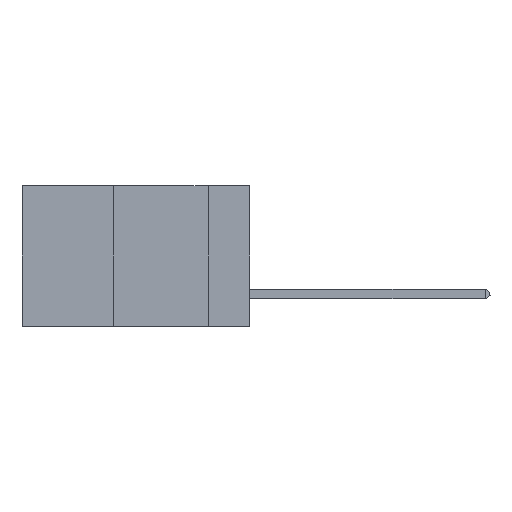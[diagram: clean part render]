
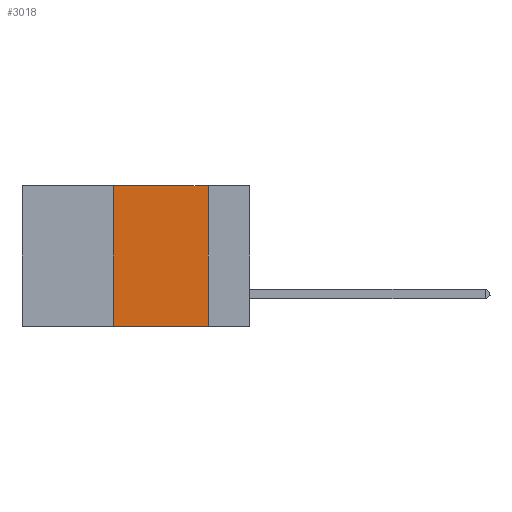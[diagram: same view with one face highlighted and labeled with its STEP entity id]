
A CAD part, left-side view. The second image highlights one B-rep face of the part: STEP entity #3018.
In plain terms, the highlighted planar face has unit normal (-1, 0, 0).
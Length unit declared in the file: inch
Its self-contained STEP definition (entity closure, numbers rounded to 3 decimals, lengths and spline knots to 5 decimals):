
#1226 = CARTESIAN_POINT ( 'NONE',  ( 0., 0.36, -0.37 ) ) ;
#2201 = ORIENTED_EDGE ( 'NONE', *, *, #19495, .F. ) ;
#3018 = ADVANCED_FACE ( 'NONE', ( #18363 ), #25612, .F. ) ;
#3512 = CARTESIAN_POINT ( 'NONE',  ( 0., 0.11, 0. ) ) ;
#3960 = CARTESIAN_POINT ( 'NONE',  ( 0., 0.6, 0. ) ) ;
#7002 = LINE ( 'NONE', #27579, #41238 ) ;
#7338 = DIRECTION ( 'NONE',  ( 0., -1., 0. ) ) ;
#7457 = LINE ( 'NONE', #19322, #32576 ) ;
#8779 = ORIENTED_EDGE ( 'NONE', *, *, #45104, .T. ) ;
#9401 = DIRECTION ( 'NONE',  ( 0., -1., 0. ) ) ;
#9418 = AXIS2_PLACEMENT_3D ( 'NONE', #3960, #40113, #14275 ) ;
#12452 = ORIENTED_EDGE ( 'NONE', *, *, #36533, .F. ) ;
#14275 = DIRECTION ( 'NONE',  ( 0., 0., -1. ) ) ;
#18363 = FACE_OUTER_BOUND ( 'NONE', #40844, .T. ) ;
#19003 = DIRECTION ( 'NONE',  ( 0., 0., 1. ) ) ;
#19322 = CARTESIAN_POINT ( 'NONE',  ( 0., 0.36, 0. ) ) ;
#19495 = EDGE_CURVE ( 'NONE', #38282, #29687, #7457, .T. ) ;
#21006 = CARTESIAN_POINT ( 'NONE',  ( 0., 0.11, -0.37 ) ) ;
#25612 = PLANE ( 'NONE',  #9418 ) ;
#26482 = LINE ( 'NONE', #39075, #32237 ) ;
#27579 = CARTESIAN_POINT ( 'NONE',  ( 0., 0.6, -0.37 ) ) ;
#29160 = CARTESIAN_POINT ( 'NONE',  ( 0., 0.6, 0. ) ) ;
#29687 = VERTEX_POINT ( 'NONE', #39628 ) ;
#32237 = VECTOR ( 'NONE', #42750, 39.37008 ) ;
#32412 = VERTEX_POINT ( 'NONE', #21006 ) ;
#32539 = ORIENTED_EDGE ( 'NONE', *, *, #43682, .F. ) ;
#32576 = VECTOR ( 'NONE', #19003, 39.37008 ) ;
#33911 = LINE ( 'NONE', #29160, #36169 ) ;
#36169 = VECTOR ( 'NONE', #7338, 39.37008 ) ;
#36533 = EDGE_CURVE ( 'NONE', #29687, #42153, #33911, .T. ) ;
#38282 = VERTEX_POINT ( 'NONE', #1226 ) ;
#39075 = CARTESIAN_POINT ( 'NONE',  ( 0., 0.11, 0. ) ) ;
#39628 = CARTESIAN_POINT ( 'NONE',  ( 0., 0.36, 0. ) ) ;
#40113 = DIRECTION ( 'NONE',  ( 1., 0., 0. ) ) ;
#40844 = EDGE_LOOP ( 'NONE', ( #32539, #12452, #2201, #8779 ) ) ;
#41238 = VECTOR ( 'NONE', #9401, 39.37008 ) ;
#42153 = VERTEX_POINT ( 'NONE', #3512 ) ;
#42750 = DIRECTION ( 'NONE',  ( 0., 0., -1. ) ) ;
#43682 = EDGE_CURVE ( 'NONE', #42153, #32412, #26482, .T. ) ;
#45104 = EDGE_CURVE ( 'NONE', #38282, #32412, #7002, .T. ) ;
